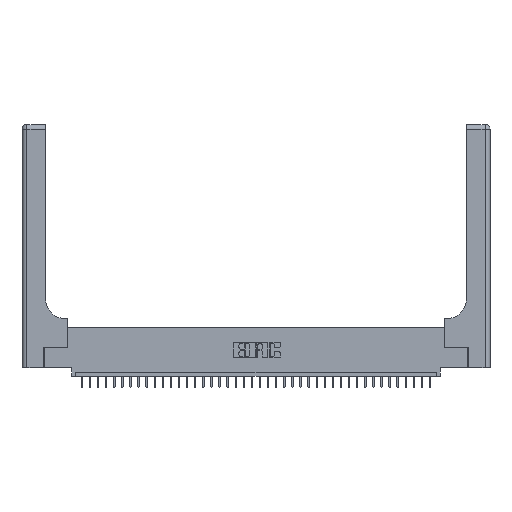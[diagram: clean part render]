
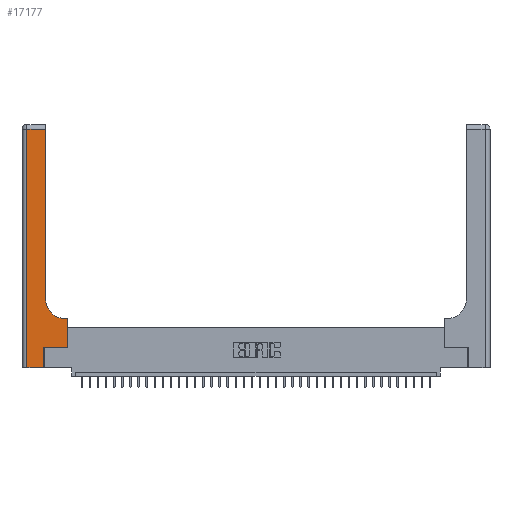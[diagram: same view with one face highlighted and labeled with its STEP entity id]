
A CAD part, top view. The second image highlights one B-rep face of the part: STEP entity #17177.
In plain terms, the highlighted planar face has unit normal (0, 0, 1).
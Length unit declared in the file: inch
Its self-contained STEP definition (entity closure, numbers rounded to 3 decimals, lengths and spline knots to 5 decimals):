
#119 = VERTEX_POINT ( 'NONE', #2941 ) ;
#432 = DIRECTION ( 'NONE',  ( -1., 0., 0. ) ) ;
#448 = ORIENTED_EDGE ( 'NONE', *, *, #23058, .T. ) ;
#496 = EDGE_CURVE ( 'NONE', #18538, #37107, #27247, .T. ) ;
#978 = EDGE_CURVE ( 'NONE', #119, #18538, #31465, .T. ) ;
#1231 = CARTESIAN_POINT ( 'NONE',  ( 0.5585, 0.25, 0.37 ) ) ;
#1380 = CARTESIAN_POINT ( 'NONE',  ( 0., 2.94, 0.37 ) ) ;
#1574 = LINE ( 'NONE', #1380, #30492 ) ;
#1951 = ORIENTED_EDGE ( 'NONE', *, *, #25948, .T. ) ;
#2107 = LINE ( 'NONE', #13310, #30060 ) ;
#2941 = CARTESIAN_POINT ( 'NONE',  ( 0.269, 0., 0.37 ) ) ;
#4093 = DIRECTION ( 'NONE',  ( -1., 0., 0. ) ) ;
#4119 = CARTESIAN_POINT ( 'NONE',  ( 0.5415, 0.85, 0.37 ) ) ;
#4297 = ORIENTED_EDGE ( 'NONE', *, *, #29654, .T. ) ;
#4800 = VERTEX_POINT ( 'NONE', #23874 ) ;
#4904 = EDGE_CURVE ( 'NONE', #27005, #26436, #8766, .T. ) ;
#5619 = EDGE_LOOP ( 'NONE', ( #1951, #35891, #22593, #4297, #18889, #12308, #448, #37138, #36459 ) ) ;
#6428 = VERTEX_POINT ( 'NONE', #35695 ) ;
#8110 = DIRECTION ( 'NONE',  ( 0., -1., 0. ) ) ;
#8368 = PLANE ( 'NONE',  #31513 ) ;
#8538 = CARTESIAN_POINT ( 'NONE',  ( 0.2915, 0.85, 0.37 ) ) ;
#8766 = CIRCLE ( 'NONE', #29145, 0.25 ) ;
#10132 = LINE ( 'NONE', #1231, #13152 ) ;
#10310 = VERTEX_POINT ( 'NONE', #20230 ) ;
#11561 = CARTESIAN_POINT ( 'NONE',  ( 0.5415, 0.6, 0.37 ) ) ;
#12010 = FACE_OUTER_BOUND ( 'NONE', #5619, .T. ) ;
#12308 = ORIENTED_EDGE ( 'NONE', *, *, #496, .T. ) ;
#13152 = VECTOR ( 'NONE', #24836, 39.37008 ) ;
#13310 = CARTESIAN_POINT ( 'NONE',  ( 0.06, 3., 0.37 ) ) ;
#13645 = CARTESIAN_POINT ( 'NONE',  ( 0.2915, 3., 0.37 ) ) ;
#14522 = DIRECTION ( 'NONE',  ( -1., 0., 0. ) ) ;
#15531 = EDGE_CURVE ( 'NONE', #6428, #27005, #21521, .T. ) ;
#17177 = ADVANCED_FACE ( 'NONE', ( #12010 ), #8368, .F. ) ;
#17912 = VECTOR ( 'NONE', #432, 39.37008 ) ;
#18538 = VERTEX_POINT ( 'NONE', #35905 ) ;
#18564 = CARTESIAN_POINT ( 'NONE',  ( 0.2915, 2.94, 0.37 ) ) ;
#18889 = ORIENTED_EDGE ( 'NONE', *, *, #978, .T. ) ;
#20230 = CARTESIAN_POINT ( 'NONE',  ( 0.06, 0., 0.37 ) ) ;
#21521 = LINE ( 'NONE', #30611, #17912 ) ;
#21533 = DIRECTION ( 'NONE',  ( 1., 0., 0. ) ) ;
#21967 = CARTESIAN_POINT ( 'NONE',  ( 0.5585, 0.25, 0.37 ) ) ;
#22593 = ORIENTED_EDGE ( 'NONE', *, *, #26806, .T. ) ;
#23058 = EDGE_CURVE ( 'NONE', #37107, #6428, #10132, .T. ) ;
#23489 = EDGE_CURVE ( 'NONE', #25246, #4800, #1574, .T. ) ;
#23874 = CARTESIAN_POINT ( 'NONE',  ( 0.06, 2.94, 0.37 ) ) ;
#23904 = CARTESIAN_POINT ( 'NONE',  ( 0., 0., 0.37 ) ) ;
#24351 = CARTESIAN_POINT ( 'NONE',  ( 0.269, 0.25, 0.37 ) ) ;
#24537 = DIRECTION ( 'NONE',  ( 1., 0., 0. ) ) ;
#24836 = DIRECTION ( 'NONE',  ( 0., 1., 0. ) ) ;
#25073 = LINE ( 'NONE', #13645, #30630 ) ;
#25246 = VERTEX_POINT ( 'NONE', #18564 ) ;
#25453 = CARTESIAN_POINT ( 'NONE',  ( 0.269, 0., 0.37 ) ) ;
#25948 = EDGE_CURVE ( 'NONE', #26436, #25246, #25073, .T. ) ;
#26436 = VERTEX_POINT ( 'NONE', #8538 ) ;
#26806 = EDGE_CURVE ( 'NONE', #4800, #10310, #2107, .T. ) ;
#27005 = VERTEX_POINT ( 'NONE', #11561 ) ;
#27247 = LINE ( 'NONE', #24351, #35691 ) ;
#27690 = VECTOR ( 'NONE', #36866, 39.37008 ) ;
#27907 = DIRECTION ( 'NONE',  ( 0., 0., -1. ) ) ;
#29145 = AXIS2_PLACEMENT_3D ( 'NONE', #4119, #27907, #21533 ) ;
#29654 = EDGE_CURVE ( 'NONE', #10310, #119, #30459, .T. ) ;
#30060 = VECTOR ( 'NONE', #8110, 39.37008 ) ;
#30459 = LINE ( 'NONE', #23904, #35726 ) ;
#30492 = VECTOR ( 'NONE', #4093, 39.37008 ) ;
#30611 = CARTESIAN_POINT ( 'NONE',  ( 0.2915, 0.6, 0.37 ) ) ;
#30630 = VECTOR ( 'NONE', #36873, 39.37008 ) ;
#31465 = LINE ( 'NONE', #25453, #27690 ) ;
#31513 = AXIS2_PLACEMENT_3D ( 'NONE', #31982, #35246, #14522 ) ;
#31982 = CARTESIAN_POINT ( 'NONE',  ( 0., 3., 0.37 ) ) ;
#32809 = DIRECTION ( 'NONE',  ( 1., 0., 0. ) ) ;
#35246 = DIRECTION ( 'NONE',  ( 0., 0., -1. ) ) ;
#35691 = VECTOR ( 'NONE', #24537, 39.37008 ) ;
#35695 = CARTESIAN_POINT ( 'NONE',  ( 0.5585, 0.6, 0.37 ) ) ;
#35726 = VECTOR ( 'NONE', #32809, 39.37008 ) ;
#35891 = ORIENTED_EDGE ( 'NONE', *, *, #23489, .T. ) ;
#35905 = CARTESIAN_POINT ( 'NONE',  ( 0.269, 0.25, 0.37 ) ) ;
#36459 = ORIENTED_EDGE ( 'NONE', *, *, #4904, .T. ) ;
#36866 = DIRECTION ( 'NONE',  ( 0., 1., 0. ) ) ;
#36873 = DIRECTION ( 'NONE',  ( 0., 1., 0. ) ) ;
#37107 = VERTEX_POINT ( 'NONE', #21967 ) ;
#37138 = ORIENTED_EDGE ( 'NONE', *, *, #15531, .T. ) ;
